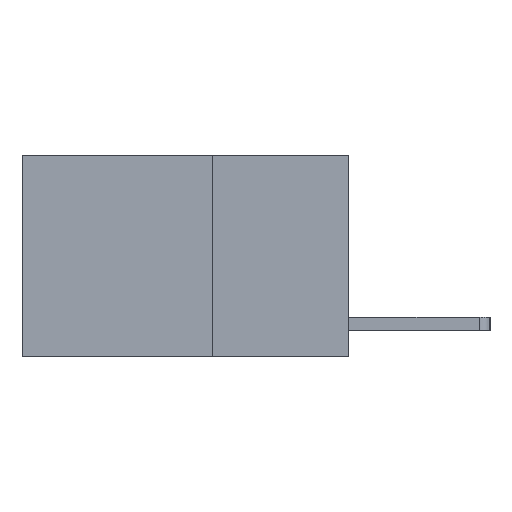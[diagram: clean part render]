
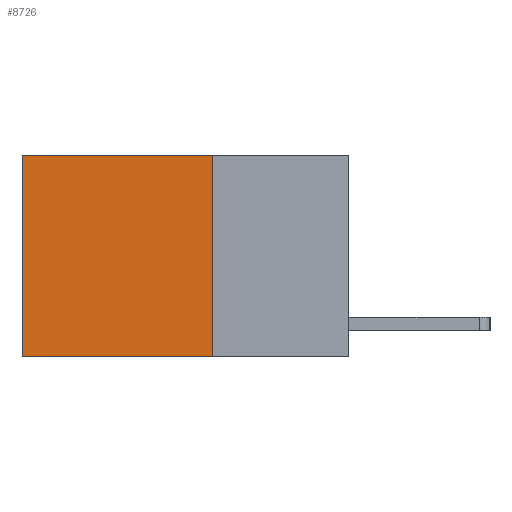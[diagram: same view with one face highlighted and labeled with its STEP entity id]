
A CAD part, left-side view. The second image highlights one B-rep face of the part: STEP entity #8726.
In plain terms, the highlighted planar face has unit normal (-1, 0, 0).
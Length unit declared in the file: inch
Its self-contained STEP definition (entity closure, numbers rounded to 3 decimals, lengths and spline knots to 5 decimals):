
#66 = EDGE_LOOP ( 'NONE', ( #7386, #9184, #3926, #590 ) ) ;
#67 = VECTOR ( 'NONE', #261, 39.37008 ) ;
#261 = DIRECTION ( 'NONE',  ( 0., 1., 0. ) ) ;
#299 = DIRECTION ( 'NONE',  ( 0., 0., -1. ) ) ;
#590 = ORIENTED_EDGE ( 'NONE', *, *, #9917, .T. ) ;
#943 = VECTOR ( 'NONE', #1949, 39.37008 ) ;
#1016 = VERTEX_POINT ( 'NONE', #7067 ) ;
#1154 = EDGE_CURVE ( 'NONE', #8776, #9635, #7168, .T. ) ;
#1694 = VECTOR ( 'NONE', #2162, 39.37008 ) ;
#1949 = DIRECTION ( 'NONE',  ( 0., 0., -1. ) ) ;
#2005 = CARTESIAN_POINT ( 'NONE',  ( 0.2625, 0.6, 0. ) ) ;
#2162 = DIRECTION ( 'NONE',  ( 0., 1., 0. ) ) ;
#2420 = EDGE_CURVE ( 'NONE', #1016, #9372, #6156, .T. ) ;
#2693 = CARTESIAN_POINT ( 'NONE',  ( 0.2625, 0.25, 0. ) ) ;
#3551 = CARTESIAN_POINT ( 'NONE',  ( 0.2625, 0.25, 0. ) ) ;
#3576 = CARTESIAN_POINT ( 'NONE',  ( 0.2625, 0.25, -0.37 ) ) ;
#3926 = ORIENTED_EDGE ( 'NONE', *, *, #2420, .F. ) ;
#4350 = CARTESIAN_POINT ( 'NONE',  ( 0.2625, 0.25, 0. ) ) ;
#4691 = CARTESIAN_POINT ( 'NONE',  ( 0.2625, 0.6, -0.37 ) ) ;
#5070 = EDGE_CURVE ( 'NONE', #9372, #9635, #10029, .T. ) ;
#5174 = DIRECTION ( 'NONE',  ( 1., 0., 0. ) ) ;
#6156 = LINE ( 'NONE', #4350, #10408 ) ;
#6548 = LINE ( 'NONE', #2693, #67 ) ;
#6812 = CARTESIAN_POINT ( 'NONE',  ( 0.2625, 0.6, 0. ) ) ;
#6994 = CARTESIAN_POINT ( 'NONE',  ( 0.2625, 0.25, -0.37 ) ) ;
#7067 = CARTESIAN_POINT ( 'NONE',  ( 0.2625, 0.25, 0. ) ) ;
#7168 = LINE ( 'NONE', #6812, #943 ) ;
#7386 = ORIENTED_EDGE ( 'NONE', *, *, #1154, .T. ) ;
#7563 = PLANE ( 'NONE',  #9478 ) ;
#8726 = ADVANCED_FACE ( 'NONE', ( #9577 ), #7563, .F. ) ;
#8776 = VERTEX_POINT ( 'NONE', #2005 ) ;
#9184 = ORIENTED_EDGE ( 'NONE', *, *, #5070, .F. ) ;
#9372 = VERTEX_POINT ( 'NONE', #3576 ) ;
#9478 = AXIS2_PLACEMENT_3D ( 'NONE', #3551, #5174, #299 ) ;
#9577 = FACE_OUTER_BOUND ( 'NONE', #66, .T. ) ;
#9635 = VERTEX_POINT ( 'NONE', #4691 ) ;
#9917 = EDGE_CURVE ( 'NONE', #1016, #8776, #6548, .T. ) ;
#9976 = DIRECTION ( 'NONE',  ( 0., 0., -1. ) ) ;
#10029 = LINE ( 'NONE', #6994, #1694 ) ;
#10408 = VECTOR ( 'NONE', #9976, 39.37008 ) ;
